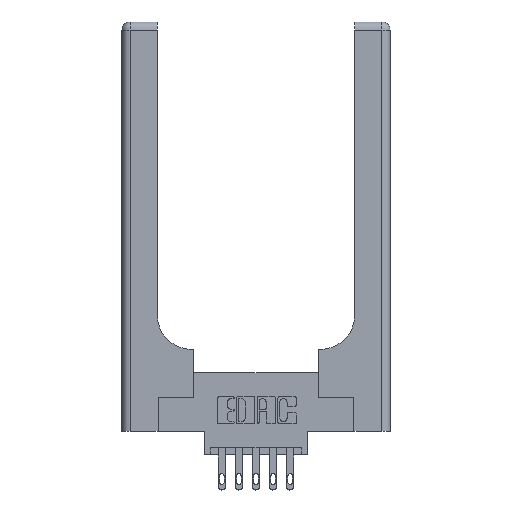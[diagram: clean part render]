
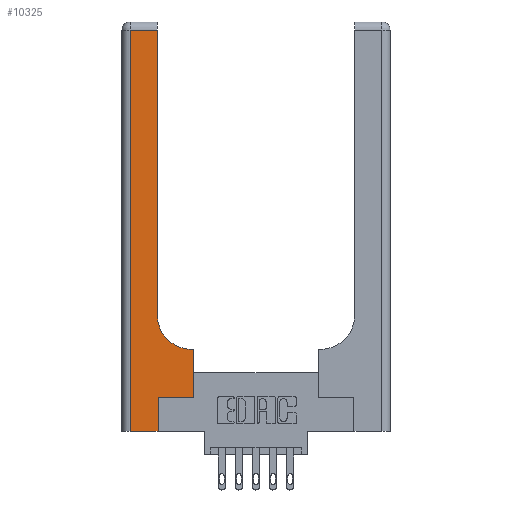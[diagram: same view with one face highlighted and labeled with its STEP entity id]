
A CAD part, top view. The second image highlights one B-rep face of the part: STEP entity #10325.
In plain terms, the highlighted planar face has unit normal (0, 0, 1).
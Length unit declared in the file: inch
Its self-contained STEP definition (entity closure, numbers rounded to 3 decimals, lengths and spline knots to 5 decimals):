
#91 = DIRECTION ( 'NONE',  ( 1., 0., 0. ) ) ;
#238 = VERTEX_POINT ( 'NONE', #8444 ) ;
#334 = DIRECTION ( 'NONE',  ( -1., 0., 0. ) ) ;
#531 = CARTESIAN_POINT ( 'NONE',  ( 0.265, 0.25, 0.37 ) ) ;
#1030 = CARTESIAN_POINT ( 'NONE',  ( 0., 0., 0.37 ) ) ;
#1463 = VECTOR ( 'NONE', #5977, 39.37008 ) ;
#1544 = LINE ( 'NONE', #7733, #9116 ) ;
#1606 = CARTESIAN_POINT ( 'NONE',  ( 0.51, 0.85, 0.37 ) ) ;
#1828 = DIRECTION ( 'NONE',  ( -1., 0., 0. ) ) ;
#1873 = ORIENTED_EDGE ( 'NONE', *, *, #3787, .T. ) ;
#1889 = CARTESIAN_POINT ( 'NONE',  ( 0.26, 0.6, 0.37 ) ) ;
#2102 = CARTESIAN_POINT ( 'NONE',  ( 0.265, 0., 0.37 ) ) ;
#2298 = ORIENTED_EDGE ( 'NONE', *, *, #8996, .T. ) ;
#2616 = ORIENTED_EDGE ( 'NONE', *, *, #5285, .T. ) ;
#2813 = ORIENTED_EDGE ( 'NONE', *, *, #13423, .T. ) ;
#2879 = LINE ( 'NONE', #2102, #8298 ) ;
#2892 = VECTOR ( 'NONE', #7482, 39.37008 ) ;
#3002 = DIRECTION ( 'NONE',  ( 0., 1., 0. ) ) ;
#3062 = LINE ( 'NONE', #1889, #8306 ) ;
#3242 = LINE ( 'NONE', #6415, #2892 ) ;
#3439 = ORIENTED_EDGE ( 'NONE', *, *, #8944, .T. ) ;
#3635 = VERTEX_POINT ( 'NONE', #6734 ) ;
#3711 = DIRECTION ( 'NONE',  ( 1., 0., 0. ) ) ;
#3787 = EDGE_CURVE ( 'NONE', #6358, #4926, #12105, .T. ) ;
#4056 = VERTEX_POINT ( 'NONE', #9832 ) ;
#4062 = LINE ( 'NONE', #4987, #1463 ) ;
#4099 = DIRECTION ( 'NONE',  ( 0., 1., 0. ) ) ;
#4187 = LINE ( 'NONE', #1030, #12056 ) ;
#4503 = VERTEX_POINT ( 'NONE', #7017 ) ;
#4597 = CARTESIAN_POINT ( 'NONE',  ( 0.265, 0., 0.37 ) ) ;
#4926 = VERTEX_POINT ( 'NONE', #9528 ) ;
#4987 = CARTESIAN_POINT ( 'NONE',  ( 0.06, 3., 0.37 ) ) ;
#5285 = EDGE_CURVE ( 'NONE', #3635, #4503, #12745, .T. ) ;
#5790 = EDGE_CURVE ( 'NONE', #4056, #7104, #4187, .T. ) ;
#5977 = DIRECTION ( 'NONE',  ( 0., -1., 0. ) ) ;
#5985 = DIRECTION ( 'NONE',  ( -1., 0., 0. ) ) ;
#6032 = AXIS2_PLACEMENT_3D ( 'NONE', #1606, #8930, #10122 ) ;
#6261 = EDGE_CURVE ( 'NONE', #12562, #238, #13756, .T. ) ;
#6358 = VERTEX_POINT ( 'NONE', #10858 ) ;
#6415 = CARTESIAN_POINT ( 'NONE',  ( 0.26, 3., 0.37 ) ) ;
#6602 = PLANE ( 'NONE',  #7331 ) ;
#6734 = CARTESIAN_POINT ( 'NONE',  ( 0.26, 2.94, 0.37 ) ) ;
#6814 = EDGE_CURVE ( 'NONE', #238, #6358, #3062, .T. ) ;
#7017 = CARTESIAN_POINT ( 'NONE',  ( 0.06, 2.94, 0.37 ) ) ;
#7104 = VERTEX_POINT ( 'NONE', #4597 ) ;
#7243 = CARTESIAN_POINT ( 'NONE',  ( 0., 2.94, 0.37 ) ) ;
#7323 = ORIENTED_EDGE ( 'NONE', *, *, #6814, .T. ) ;
#7331 = AXIS2_PLACEMENT_3D ( 'NONE', #11909, #8809, #334 ) ;
#7482 = DIRECTION ( 'NONE',  ( 0., 1., 0. ) ) ;
#7606 = ORIENTED_EDGE ( 'NONE', *, *, #5790, .T. ) ;
#7733 = CARTESIAN_POINT ( 'NONE',  ( 0.265, 0.25, 0.37 ) ) ;
#8298 = VECTOR ( 'NONE', #3002, 39.37008 ) ;
#8306 = VECTOR ( 'NONE', #1828, 39.37008 ) ;
#8444 = CARTESIAN_POINT ( 'NONE',  ( 0.528, 0.6, 0.37 ) ) ;
#8809 = DIRECTION ( 'NONE',  ( 0., 0., -1. ) ) ;
#8930 = DIRECTION ( 'NONE',  ( 0., 0., -1. ) ) ;
#8944 = EDGE_CURVE ( 'NONE', #11962, #12562, #1544, .T. ) ;
#8996 = EDGE_CURVE ( 'NONE', #4503, #4056, #4062, .T. ) ;
#9116 = VECTOR ( 'NONE', #3711, 39.37008 ) ;
#9528 = CARTESIAN_POINT ( 'NONE',  ( 0.26, 0.85, 0.37 ) ) ;
#9741 = CARTESIAN_POINT ( 'NONE',  ( 0.528, 0.25, 0.37 ) ) ;
#9832 = CARTESIAN_POINT ( 'NONE',  ( 0.06, 0., 0.37 ) ) ;
#9834 = ORIENTED_EDGE ( 'NONE', *, *, #13702, .T. ) ;
#10122 = DIRECTION ( 'NONE',  ( 1., 0., 0. ) ) ;
#10128 = VECTOR ( 'NONE', #4099, 39.37008 ) ;
#10325 = ADVANCED_FACE ( 'NONE', ( #11980 ), #6602, .F. ) ;
#10684 = VECTOR ( 'NONE', #5985, 39.37008 ) ;
#10858 = CARTESIAN_POINT ( 'NONE',  ( 0.51, 0.6, 0.37 ) ) ;
#11579 = CARTESIAN_POINT ( 'NONE',  ( 0.528, 0.25, 0.37 ) ) ;
#11909 = CARTESIAN_POINT ( 'NONE',  ( 0., 3., 0.37 ) ) ;
#11962 = VERTEX_POINT ( 'NONE', #531 ) ;
#11980 = FACE_OUTER_BOUND ( 'NONE', #12104, .T. ) ;
#12056 = VECTOR ( 'NONE', #91, 39.37008 ) ;
#12104 = EDGE_LOOP ( 'NONE', ( #9834, #2616, #2298, #7606, #2813, #3439, #12890, #7323, #1873 ) ) ;
#12105 = CIRCLE ( 'NONE', #6032, 0.25 ) ;
#12562 = VERTEX_POINT ( 'NONE', #9741 ) ;
#12745 = LINE ( 'NONE', #7243, #10684 ) ;
#12890 = ORIENTED_EDGE ( 'NONE', *, *, #6261, .T. ) ;
#13423 = EDGE_CURVE ( 'NONE', #7104, #11962, #2879, .T. ) ;
#13702 = EDGE_CURVE ( 'NONE', #4926, #3635, #3242, .T. ) ;
#13756 = LINE ( 'NONE', #11579, #10128 ) ;
